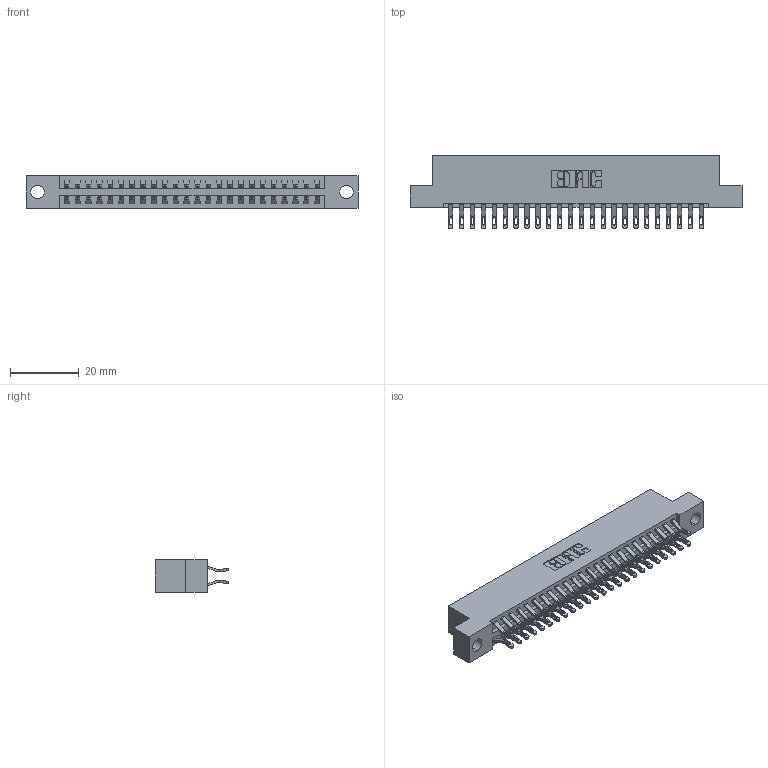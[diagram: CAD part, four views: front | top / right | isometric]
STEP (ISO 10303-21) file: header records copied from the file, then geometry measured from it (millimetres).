
FILE_DESCRIPTION (( 'STEP AP203' ), '1' );
FILE_NAME ('346-048-555-204.STEP', '2018-08-25T10:26:06', ( '' ), ( '' ), 'SwSTEP 2.0', 'SolidWorks 2016', '' );
FILE_SCHEMA (( 'CONFIG_CONTROL_DESIGN' ));
Length unit declared in the file: inch
Products named in the file (3): 345-292-001_555 Tail; 346-048-555-204; 346 Part_Flush Mounting Lugs - 0.156 Dia-TH
Assembly tree (49 placements, depth 2):
  346-048-555-204
    346 Part_Flush Mounting Lugs - 0.156 Dia-TH
    345-292-001_555 Tail  x48
Bounding box: 96.77 x 21.46 x 9.4 mm (x, y, z)
Volume: 9348.2 mm3; surface area: 12876.5 mm2
Topology: 49 solids, 49 shells, 2906 faces, 9113 edges, 6074 vertices
Faces by surface type: plane 1660, cylinder 1246
Entity records: 18415 total; most frequent: CARTESIAN_POINT 3094, ORIENTED_EDGE 2998, DIRECTION 2747, EDGE_CURVE 1499, VECTOR 1251, LINE 1251, VERTEX_POINT 998, AXIS2_PLACEMENT_3D 748
